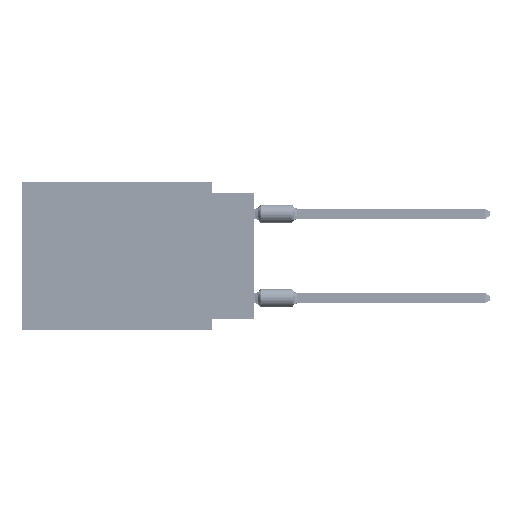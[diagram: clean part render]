
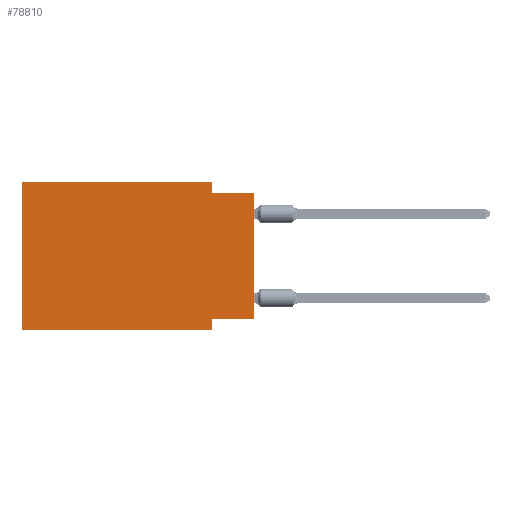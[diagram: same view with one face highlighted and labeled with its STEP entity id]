
A CAD part, left-side view. The second image highlights one B-rep face of the part: STEP entity #78810.
In plain terms, the highlighted planar face has unit normal (-1, 0, 0).
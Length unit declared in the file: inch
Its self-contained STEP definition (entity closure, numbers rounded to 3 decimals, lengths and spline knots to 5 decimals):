
#752 = VERTEX_POINT ( 'NONE', #33913 ) ;
#3037 = CARTESIAN_POINT ( 'NONE',  ( 0., 0.1, -0.325 ) ) ;
#4885 = CARTESIAN_POINT ( 'NONE',  ( 0., 0.1, 0. ) ) ;
#5900 = CARTESIAN_POINT ( 'NONE',  ( 0., 0.1, -0.35 ) ) ;
#5937 = EDGE_CURVE ( 'NONE', #32060, #50733, #37742, .T. ) ;
#6138 = VECTOR ( 'NONE', #63944, 39.37008 ) ;
#9010 = ORIENTED_EDGE ( 'NONE', *, *, #5937, .F. ) ;
#9448 = EDGE_CURVE ( 'NONE', #90176, #45762, #82778, .T. ) ;
#9713 = CARTESIAN_POINT ( 'NONE',  ( 0., 0.55, 0. ) ) ;
#24602 = DIRECTION ( 'NONE',  ( 0., -1., 0. ) ) ;
#28490 = EDGE_CURVE ( 'NONE', #752, #32060, #77710, .T. ) ;
#30933 = DIRECTION ( 'NONE',  ( 0., 1., 0. ) ) ;
#32060 = VERTEX_POINT ( 'NONE', #3037 ) ;
#33848 = CARTESIAN_POINT ( 'NONE',  ( 0., 0.55, 0. ) ) ;
#33913 = CARTESIAN_POINT ( 'NONE',  ( 0., 0., -0.325 ) ) ;
#34487 = FACE_OUTER_BOUND ( 'NONE', #59831, .T. ) ;
#36271 = VERTEX_POINT ( 'NONE', #9713 ) ;
#37742 = LINE ( 'NONE', #48810, #79313 ) ;
#41889 = DIRECTION ( 'NONE',  ( 1., 0., 0. ) ) ;
#44463 = VERTEX_POINT ( 'NONE', #48002 ) ;
#45090 = DIRECTION ( 'NONE',  ( 0., 0., 1. ) ) ;
#45762 = VERTEX_POINT ( 'NONE', #90996 ) ;
#47588 = EDGE_CURVE ( 'NONE', #44463, #36271, #111140, .T. ) ;
#48002 = CARTESIAN_POINT ( 'NONE',  ( 0., 0.55, -0.35 ) ) ;
#48810 = CARTESIAN_POINT ( 'NONE',  ( 0., 0.1, -0.35 ) ) ;
#49380 = CARTESIAN_POINT ( 'NONE',  ( 0., 0., -0.325 ) ) ;
#50733 = VERTEX_POINT ( 'NONE', #5900 ) ;
#55244 = ORIENTED_EDGE ( 'NONE', *, *, #9448, .F. ) ;
#56551 = CARTESIAN_POINT ( 'NONE',  ( 0., 0.1, -0.025 ) ) ;
#59664 = CARTESIAN_POINT ( 'NONE',  ( 0., 0.1, 0. ) ) ;
#59831 = EDGE_LOOP ( 'NONE', ( #100579, #55244, #110046, #101949, #114302, #61876, #9010, #117871 ) ) ;
#61876 = ORIENTED_EDGE ( 'NONE', *, *, #101406, .T. ) ;
#63321 = VERTEX_POINT ( 'NONE', #59664 ) ;
#63944 = DIRECTION ( 'NONE',  ( 0., -1., 0. ) ) ;
#64695 = VECTOR ( 'NONE', #30933, 39.37008 ) ;
#64838 = AXIS2_PLACEMENT_3D ( 'NONE', #109582, #41889, #99777 ) ;
#69647 = VECTOR ( 'NONE', #45090, 39.37008 ) ;
#71694 = EDGE_CURVE ( 'NONE', #752, #45762, #109750, .T. ) ;
#72658 = PLANE ( 'NONE',  #64838 ) ;
#73808 = LINE ( 'NONE', #94684, #6138 ) ;
#73814 = LINE ( 'NONE', #33848, #91899 ) ;
#77710 = LINE ( 'NONE', #49380, #64695 ) ;
#78810 = ADVANCED_FACE ( 'NONE', ( #34487 ), #72658, .F. ) ;
#79313 = VECTOR ( 'NONE', #105435, 39.37008 ) ;
#79629 = VECTOR ( 'NONE', #117905, 39.37008 ) ;
#80534 = VECTOR ( 'NONE', #93907, 39.37008 ) ;
#82778 = LINE ( 'NONE', #118503, #79629 ) ;
#89255 = LINE ( 'NONE', #4885, #110375 ) ;
#90176 = VERTEX_POINT ( 'NONE', #56551 ) ;
#90996 = CARTESIAN_POINT ( 'NONE',  ( 0., 0., -0.025 ) ) ;
#91899 = VECTOR ( 'NONE', #24602, 39.37008 ) ;
#93907 = DIRECTION ( 'NONE',  ( 0., 0., 1. ) ) ;
#94684 = CARTESIAN_POINT ( 'NONE',  ( 0., 0.55, -0.35 ) ) ;
#99777 = DIRECTION ( 'NONE',  ( 0., 0., -1. ) ) ;
#100579 = ORIENTED_EDGE ( 'NONE', *, *, #71694, .T. ) ;
#101298 = EDGE_CURVE ( 'NONE', #63321, #90176, #89255, .T. ) ;
#101406 = EDGE_CURVE ( 'NONE', #44463, #50733, #73808, .T. ) ;
#101744 = CARTESIAN_POINT ( 'NONE',  ( 0., 0., 0. ) ) ;
#101949 = ORIENTED_EDGE ( 'NONE', *, *, #114159, .F. ) ;
#105435 = DIRECTION ( 'NONE',  ( 0., 0., -1. ) ) ;
#108923 = DIRECTION ( 'NONE',  ( 0., 0., -1. ) ) ;
#109582 = CARTESIAN_POINT ( 'NONE',  ( 0., 0.55, 0. ) ) ;
#109750 = LINE ( 'NONE', #101744, #69647 ) ;
#110046 = ORIENTED_EDGE ( 'NONE', *, *, #101298, .F. ) ;
#110375 = VECTOR ( 'NONE', #108923, 39.37008 ) ;
#111140 = LINE ( 'NONE', #121599, #80534 ) ;
#114159 = EDGE_CURVE ( 'NONE', #36271, #63321, #73814, .T. ) ;
#114302 = ORIENTED_EDGE ( 'NONE', *, *, #47588, .F. ) ;
#117871 = ORIENTED_EDGE ( 'NONE', *, *, #28490, .F. ) ;
#117905 = DIRECTION ( 'NONE',  ( 0., -1., 0. ) ) ;
#118503 = CARTESIAN_POINT ( 'NONE',  ( 0., 0., -0.025 ) ) ;
#121599 = CARTESIAN_POINT ( 'NONE',  ( 0., 0.55, 0. ) ) ;
